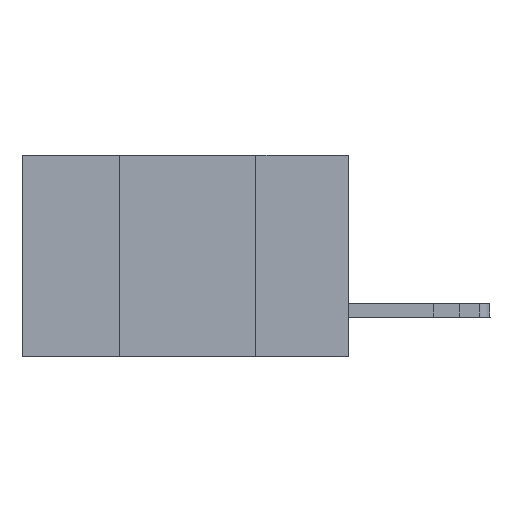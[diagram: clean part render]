
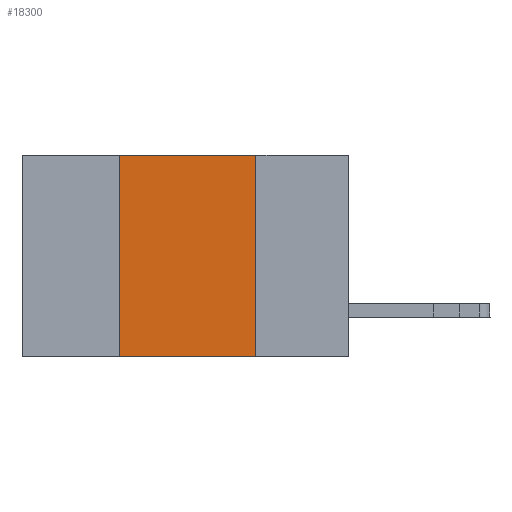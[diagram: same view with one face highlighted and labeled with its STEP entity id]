
A CAD part, left-side view. The second image highlights one B-rep face of the part: STEP entity #18300.
In plain terms, the highlighted planar face has unit normal (-1, 0, 0).
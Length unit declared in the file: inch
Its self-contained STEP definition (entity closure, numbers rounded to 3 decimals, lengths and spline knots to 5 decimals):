
#189 = CARTESIAN_POINT ( 'NONE',  ( 0., 0.42, 0. ) ) ;
#999 = FACE_OUTER_BOUND ( 'NONE', #17087, .T. ) ;
#1067 = VECTOR ( 'NONE', #21975, 39.37008 ) ;
#1319 = LINE ( 'NONE', #12010, #1067 ) ;
#1665 = LINE ( 'NONE', #189, #9958 ) ;
#1722 = CARTESIAN_POINT ( 'NONE',  ( 0., 0.6, -0.37 ) ) ;
#3065 = AXIS2_PLACEMENT_3D ( 'NONE', #13813, #15529, #17150 ) ;
#3513 = LINE ( 'NONE', #12815, #6719 ) ;
#3534 = EDGE_CURVE ( 'NONE', #5898, #4224, #1665, .T. ) ;
#4224 = VERTEX_POINT ( 'NONE', #15944 ) ;
#5257 = PLANE ( 'NONE',  #3065 ) ;
#5263 = VECTOR ( 'NONE', #8445, 39.37008 ) ;
#5898 = VERTEX_POINT ( 'NONE', #12613 ) ;
#6472 = CARTESIAN_POINT ( 'NONE',  ( 0., 0.17, 0. ) ) ;
#6719 = VECTOR ( 'NONE', #11033, 39.37008 ) ;
#8445 = DIRECTION ( 'NONE',  ( 0., -1., 0. ) ) ;
#9821 = EDGE_CURVE ( 'NONE', #18067, #15515, #3513, .T. ) ;
#9958 = VECTOR ( 'NONE', #15553, 39.37008 ) ;
#10095 = ORIENTED_EDGE ( 'NONE', *, *, #9821, .F. ) ;
#10744 = ORIENTED_EDGE ( 'NONE', *, *, #16678, .T. ) ;
#10775 = ORIENTED_EDGE ( 'NONE', *, *, #15628, .F. ) ;
#11033 = DIRECTION ( 'NONE',  ( 0., 0., -1. ) ) ;
#12010 = CARTESIAN_POINT ( 'NONE',  ( 0., 0.6, 0. ) ) ;
#12613 = CARTESIAN_POINT ( 'NONE',  ( 0., 0.42, -0.37 ) ) ;
#12815 = CARTESIAN_POINT ( 'NONE',  ( 0., 0.17, 0. ) ) ;
#13813 = CARTESIAN_POINT ( 'NONE',  ( 0., 0.6, 0. ) ) ;
#15515 = VERTEX_POINT ( 'NONE', #16088 ) ;
#15529 = DIRECTION ( 'NONE',  ( 1., 0., 0. ) ) ;
#15553 = DIRECTION ( 'NONE',  ( 0., 0., 1. ) ) ;
#15628 = EDGE_CURVE ( 'NONE', #4224, #18067, #1319, .T. ) ;
#15944 = CARTESIAN_POINT ( 'NONE',  ( 0., 0.42, 0. ) ) ;
#16088 = CARTESIAN_POINT ( 'NONE',  ( 0., 0.17, -0.37 ) ) ;
#16678 = EDGE_CURVE ( 'NONE', #5898, #15515, #19931, .T. ) ;
#17087 = EDGE_LOOP ( 'NONE', ( #10095, #10775, #17684, #10744 ) ) ;
#17150 = DIRECTION ( 'NONE',  ( 0., 0., -1. ) ) ;
#17684 = ORIENTED_EDGE ( 'NONE', *, *, #3534, .F. ) ;
#18067 = VERTEX_POINT ( 'NONE', #6472 ) ;
#18300 = ADVANCED_FACE ( 'NONE', ( #999 ), #5257, .F. ) ;
#19931 = LINE ( 'NONE', #1722, #5263 ) ;
#21975 = DIRECTION ( 'NONE',  ( 0., -1., 0. ) ) ;
